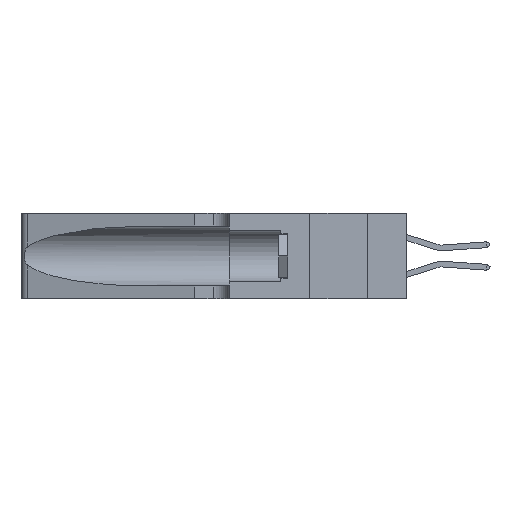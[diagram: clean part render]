
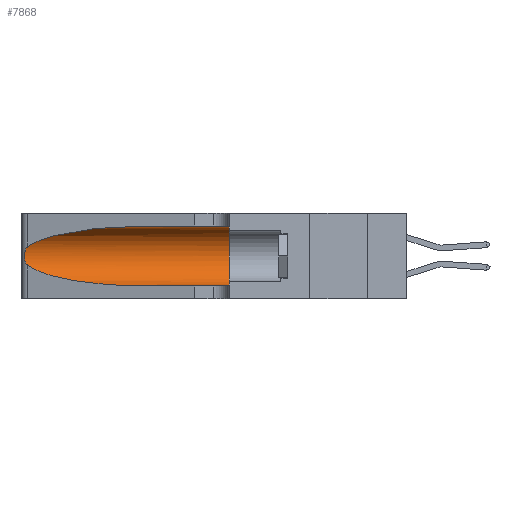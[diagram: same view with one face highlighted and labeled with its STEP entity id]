
A CAD part, left-side view. The second image highlights one B-rep face of the part: STEP entity #7868.
In plain terms, the highlighted cylindrical face has radius 3.308 mm (diameter 6.617 mm), a partial arc.
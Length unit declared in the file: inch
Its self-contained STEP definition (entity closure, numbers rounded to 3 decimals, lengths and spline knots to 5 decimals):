
#604 = CARTESIAN_POINT ( 'NONE',  ( 0.25639, 1.23186, 0.15144 ) ) ;
#973 = CARTESIAN_POINT ( 'NONE',  ( 0.1305, 0.72297, 0.05475 ) ) ;
#4133 = LINE ( 'NONE', #14661, #5261 ) ;
#4173 = CARTESIAN_POINT ( 'NONE',  ( 0.25487, 1.22718, 0.14631 ) ) ;
#5261 = VECTOR ( 'NONE', #11081, 39.37008 ) ;
#7356 =( BOUNDED_CURVE ( )  B_SPLINE_CURVE ( 3, ( #36244, #39649, #22287, #973 ),
 .UNSPECIFIED., .F., .F. ) 
 B_SPLINE_CURVE_WITH_KNOTS ( ( 4, 4 ),
 ( 3.44316, 4.71239 ),
 .UNSPECIFIED. ) 
 CURVE ( )  GEOMETRIC_REPRESENTATION_ITEM ( )  RATIONAL_B_SPLINE_CURVE ( ( 1., 0.87, 0.87, 1. ) ) 
 REPRESENTATION_ITEM ( '' )  );
#7398 = EDGE_CURVE ( 'NONE', #25497, #17155, #27280, .T. ) ;
#7400 = VERTEX_POINT ( 'NONE', #9742 ) ;
#7596 = CARTESIAN_POINT ( 'NONE',  ( 0.25639, 1.23184, 0.21858 ) ) ;
#7868 = ADVANCED_FACE ( 'NONE', ( #17767 ), #43685, .F. ) ;
#9587 = CARTESIAN_POINT ( 'NONE',  ( 0.2373, 1.15595, 0.28018 ) ) ;
#9742 = CARTESIAN_POINT ( 'NONE',  ( 0.1305, 0.72297, 0.05475 ) ) ;
#9979 = ORIENTED_EDGE ( 'NONE', *, *, #40356, .F. ) ;
#11081 = DIRECTION ( 'NONE',  ( 0., -1., 0. ) ) ;
#11163 = CARTESIAN_POINT ( 'NONE',  ( 0.25854, 1.2359, 0.20912 ) ) ;
#11365 = CARTESIAN_POINT ( 'NONE',  ( 0.25487, 1.22718, 0.22369 ) ) ;
#12356 = ORIENTED_EDGE ( 'NONE', *, *, #37978, .T. ) ;
#12830 = DIRECTION ( 'NONE',  ( 0., -1., 0. ) ) ;
#14581 = CARTESIAN_POINT ( 'NONE',  ( 0.25555, 1.22994, 0.2215 ) ) ;
#14661 = CARTESIAN_POINT ( 'NONE',  ( 0.1305, 1.61858, 0.05475 ) ) ;
#14749 = CARTESIAN_POINT ( 'NONE',  ( 0.26075, 1.23896, 0.19203 ) ) ;
#15101 = DIRECTION ( 'NONE',  ( 0., 1., 0. ) ) ;
#15627 = B_SPLINE_CURVE_WITH_KNOTS ( 'NONE', 3,
 ( #28674, #14581, #7596, #32299, #11163, #35881, #14749, #39423, #18327, #42949, #21910, #604, #25468, #4173 ),
 .UNSPECIFIED., .F., .F.,
 ( 4, 2, 2, 2, 2, 2, 4 ),
 ( 0., 0.00027, 0.00053, 0.00107, 0.0016, 0.00187, 0.00214 ),
 .UNSPECIFIED. ) ;
#15971 = CARTESIAN_POINT ( 'NONE',  ( 0.1305, 1.61858, 0.31525 ) ) ;
#16136 = LINE ( 'NONE', #15971, #44252 ) ;
#16414 = CARTESIAN_POINT ( 'NONE',  ( 0.1305, 1.61858, 0.185 ) ) ;
#16673 = CARTESIAN_POINT ( 'NONE',  ( 0.1305, 0.72297, 0.31525 ) ) ;
#16760 = CARTESIAN_POINT ( 'NONE',  ( 0.18966, 0.96281, 0.31525 ) ) ;
#17155 = VERTEX_POINT ( 'NONE', #11365 ) ;
#17767 = FACE_OUTER_BOUND ( 'NONE', #38967, .T. ) ;
#18327 = CARTESIAN_POINT ( 'NONE',  ( 0.26017, 1.23833, 0.17102 ) ) ;
#18415 = ORIENTED_EDGE ( 'NONE', *, *, #31086, .T. ) ;
#19570 = DIRECTION ( 'NONE',  ( 0., -1., 0. ) ) ;
#20348 = CARTESIAN_POINT ( 'NONE',  ( 0.1305, 0.72297, 0.31525 ) ) ;
#21660 = CARTESIAN_POINT ( 'NONE',  ( 0.1305, 0.35, 0.31525 ) ) ;
#21780 = ORIENTED_EDGE ( 'NONE', *, *, #7398, .T. ) ;
#21910 = CARTESIAN_POINT ( 'NONE',  ( 0.25789, 1.23486, 0.15765 ) ) ;
#22287 = CARTESIAN_POINT ( 'NONE',  ( 0.18966, 0.96281, 0.05475 ) ) ;
#23870 = EDGE_CURVE ( 'NONE', #17155, #28474, #15627, .T. ) ;
#23912 = CARTESIAN_POINT ( 'NONE',  ( 0.25487, 1.22718, 0.22369 ) ) ;
#25468 = CARTESIAN_POINT ( 'NONE',  ( 0.25555, 1.22993, 0.14849 ) ) ;
#25497 = VERTEX_POINT ( 'NONE', #16673 ) ;
#27280 =( BOUNDED_CURVE ( )  B_SPLINE_CURVE ( 3, ( #20348, #16760, #9587, #23912 ),
 .UNSPECIFIED., .F., .F. ) 
 B_SPLINE_CURVE_WITH_KNOTS ( ( 4, 4 ),
 ( 1.5708, 2.84003 ),
 .UNSPECIFIED. ) 
 CURVE ( )  GEOMETRIC_REPRESENTATION_ITEM ( )  RATIONAL_B_SPLINE_CURVE ( ( 1., 0.87, 0.87, 1. ) ) 
 REPRESENTATION_ITEM ( '' )  );
#27592 = VERTEX_POINT ( 'NONE', #36993 ) ;
#28474 = VERTEX_POINT ( 'NONE', #35060 ) ;
#28674 = CARTESIAN_POINT ( 'NONE',  ( 0.25487, 1.22718, 0.22369 ) ) ;
#30721 = ORIENTED_EDGE ( 'NONE', *, *, #23870, .T. ) ;
#31086 = EDGE_CURVE ( 'NONE', #28474, #7400, #7356, .T. ) ;
#32299 = CARTESIAN_POINT ( 'NONE',  ( 0.25787, 1.23484, 0.2124 ) ) ;
#33348 = AXIS2_PLACEMENT_3D ( 'NONE', #36220, #15101, #39783 ) ;
#33787 = AXIS2_PLACEMENT_3D ( 'NONE', #16414, #12830, #37530 ) ;
#35060 = CARTESIAN_POINT ( 'NONE',  ( 0.25487, 1.22718, 0.14631 ) ) ;
#35881 = CARTESIAN_POINT ( 'NONE',  ( 0.26018, 1.23835, 0.19895 ) ) ;
#36220 = CARTESIAN_POINT ( 'NONE',  ( 0.1305, 0.35, 0.185 ) ) ;
#36244 = CARTESIAN_POINT ( 'NONE',  ( 0.25487, 1.22718, 0.14631 ) ) ;
#36993 = CARTESIAN_POINT ( 'NONE',  ( 0.1305, 0.35, 0.05475 ) ) ;
#37530 = DIRECTION ( 'NONE',  ( 0., 0., -1. ) ) ;
#37978 = EDGE_CURVE ( 'NONE', #7400, #27592, #4133, .T. ) ;
#38967 = EDGE_LOOP ( 'NONE', ( #21780, #30721, #18415, #12356, #43299, #9979 ) ) ;
#39423 = CARTESIAN_POINT ( 'NONE',  ( 0.26075, 1.23896, 0.178 ) ) ;
#39649 = CARTESIAN_POINT ( 'NONE',  ( 0.2373, 1.15595, 0.08982 ) ) ;
#39783 = DIRECTION ( 'NONE',  ( 0., 0., 1. ) ) ;
#40356 = EDGE_CURVE ( 'NONE', #25497, #45199, #16136, .T. ) ;
#42949 = CARTESIAN_POINT ( 'NONE',  ( 0.25856, 1.23593, 0.16098 ) ) ;
#43299 = ORIENTED_EDGE ( 'NONE', *, *, #45320, .F. ) ;
#43685 = CYLINDRICAL_SURFACE ( 'NONE', #33787, 0.13025 ) ;
#44252 = VECTOR ( 'NONE', #19570, 39.37008 ) ;
#44884 = CIRCLE ( 'NONE', #33348, 0.13025 ) ;
#45199 = VERTEX_POINT ( 'NONE', #21660 ) ;
#45320 = EDGE_CURVE ( 'NONE', #45199, #27592, #44884, .T. ) ;
